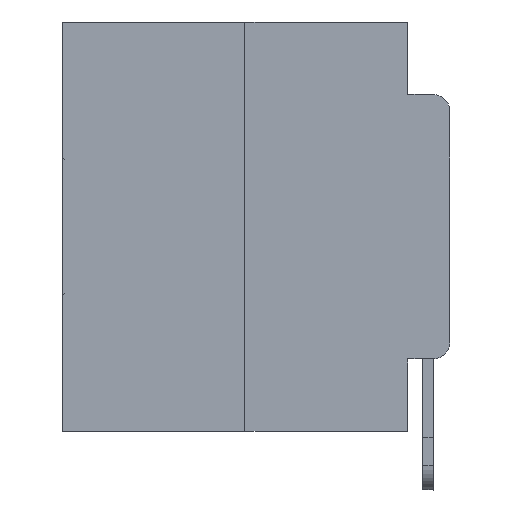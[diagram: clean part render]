
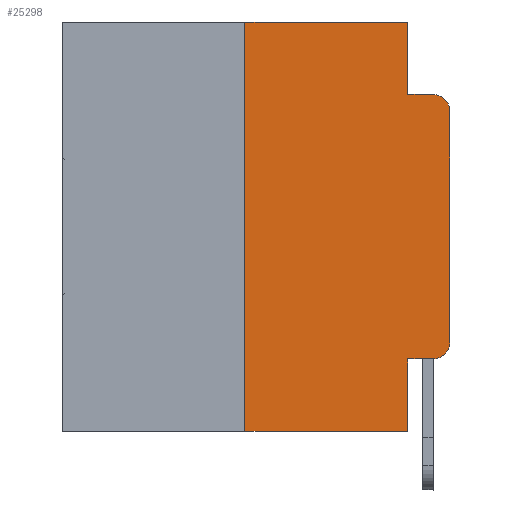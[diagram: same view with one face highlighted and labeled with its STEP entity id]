
A CAD part, left-side view. The second image highlights one B-rep face of the part: STEP entity #25298.
In plain terms, the highlighted planar face has unit normal (-1, 0, 0).
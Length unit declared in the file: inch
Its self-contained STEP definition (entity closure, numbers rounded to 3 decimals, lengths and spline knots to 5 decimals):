
#130 = VECTOR ( 'NONE', #13997, 39.37008 ) ;
#532 = ORIENTED_EDGE ( 'NONE', *, *, #11982, .T. ) ;
#886 = EDGE_CURVE ( 'NONE', #19352, #8026, #24660, .T. ) ;
#1176 = CARTESIAN_POINT ( 'NONE',  ( 0., 0.473, 0. ) ) ;
#1223 = CARTESIAN_POINT ( 'NONE',  ( 0., 0., -0.1085 ) ) ;
#1340 = LINE ( 'NONE', #13745, #18940 ) ;
#2053 = ORIENTED_EDGE ( 'NONE', *, *, #2154, .F. ) ;
#2087 = VECTOR ( 'NONE', #6164, 39.37008 ) ;
#2154 = EDGE_CURVE ( 'NONE', #3891, #13983, #21963, .T. ) ;
#2384 = ORIENTED_EDGE ( 'NONE', *, *, #26348, .F. ) ;
#3528 = DIRECTION ( 'NONE',  ( -1., 0., 0. ) ) ;
#3891 = VERTEX_POINT ( 'NONE', #13597 ) ;
#3935 = DIRECTION ( 'NONE',  ( 0., -1., 0. ) ) ;
#4432 = LINE ( 'NONE', #24332, #28053 ) ;
#5419 = ORIENTED_EDGE ( 'NONE', *, *, #17209, .F. ) ;
#6070 = CARTESIAN_POINT ( 'NONE',  ( 0., 0., 0. ) ) ;
#6164 = DIRECTION ( 'NONE',  ( 0., 0., 1. ) ) ;
#6978 = CARTESIAN_POINT ( 'NONE',  ( 0., 0.02, -0.4115 ) ) ;
#7017 = EDGE_CURVE ( 'NONE', #18324, #24548, #26638, .T. ) ;
#7060 = CARTESIAN_POINT ( 'NONE',  ( 0., 0.051, -0.0885 ) ) ;
#7067 = CARTESIAN_POINT ( 'NONE',  ( 0., 0.051, 0. ) ) ;
#8026 = VERTEX_POINT ( 'NONE', #6978 ) ;
#8273 = CARTESIAN_POINT ( 'NONE',  ( 0., 0.051, 0. ) ) ;
#8702 = ORIENTED_EDGE ( 'NONE', *, *, #23563, .T. ) ;
#9861 = CARTESIAN_POINT ( 'NONE',  ( 0., 0.02, -0.0885 ) ) ;
#9967 = ORIENTED_EDGE ( 'NONE', *, *, #7017, .T. ) ;
#10053 = VECTOR ( 'NONE', #12618, 39.37008 ) ;
#10339 = EDGE_CURVE ( 'NONE', #19352, #19735, #18447, .T. ) ;
#10655 = EDGE_LOOP ( 'NONE', ( #532, #9967, #29059, #2053, #5419, #2384, #21065, #13133, #23155, #8702 ) ) ;
#11982 = EDGE_CURVE ( 'NONE', #29237, #18324, #27941, .T. ) ;
#12618 = DIRECTION ( 'NONE',  ( 0., 0., 1. ) ) ;
#12788 = AXIS2_PLACEMENT_3D ( 'NONE', #14860, #3528, #26410 ) ;
#12840 = DIRECTION ( 'NONE',  ( 0., -1., 0. ) ) ;
#12904 = DIRECTION ( 'NONE',  ( 0., -1., 0. ) ) ;
#13133 = ORIENTED_EDGE ( 'NONE', *, *, #10339, .F. ) ;
#13396 = CARTESIAN_POINT ( 'NONE',  ( 0., 0.25, -0.5 ) ) ;
#13597 = CARTESIAN_POINT ( 'NONE',  ( 0., 0.051, 0. ) ) ;
#13680 = VERTEX_POINT ( 'NONE', #15110 ) ;
#13745 = CARTESIAN_POINT ( 'NONE',  ( 0., 0.473, -0.5 ) ) ;
#13842 = DIRECTION ( 'NONE',  ( 0., -1., 0. ) ) ;
#13864 = DIRECTION ( 'NONE',  ( 1., 0., 0. ) ) ;
#13967 = AXIS2_PLACEMENT_3D ( 'NONE', #22768, #13864, #25258 ) ;
#13983 = VERTEX_POINT ( 'NONE', #7060 ) ;
#13997 = DIRECTION ( 'NONE',  ( 0., 0., -1. ) ) ;
#14196 = EDGE_CURVE ( 'NONE', #13983, #24548, #4432, .T. ) ;
#14860 = CARTESIAN_POINT ( 'NONE',  ( 0., 0.02, -0.3915 ) ) ;
#15064 = CARTESIAN_POINT ( 'NONE',  ( 0., 0.051, -0.4115 ) ) ;
#15097 = CARTESIAN_POINT ( 'NONE',  ( 0., 0.25, 0. ) ) ;
#15110 = CARTESIAN_POINT ( 'NONE',  ( 0., 0.25, 0. ) ) ;
#15149 = VECTOR ( 'NONE', #29164, 39.37008 ) ;
#15243 = CARTESIAN_POINT ( 'NONE',  ( 0., 0.02, -0.1085 ) ) ;
#15351 = DIRECTION ( 'NONE',  ( 0., 0., -1. ) ) ;
#15655 = DIRECTION ( 'NONE',  ( -1., 0., 0. ) ) ;
#16658 = CARTESIAN_POINT ( 'NONE',  ( 0., 0.051, -0.4115 ) ) ;
#17209 = EDGE_CURVE ( 'NONE', #13680, #3891, #17599, .T. ) ;
#17599 = LINE ( 'NONE', #1176, #27919 ) ;
#17912 = FACE_OUTER_BOUND ( 'NONE', #10655, .T. ) ;
#18324 = VERTEX_POINT ( 'NONE', #1223 ) ;
#18358 = CIRCLE ( 'NONE', #12788, 0.02 ) ;
#18447 = LINE ( 'NONE', #7067, #130 ) ;
#18646 = EDGE_CURVE ( 'NONE', #20376, #19735, #1340, .T. ) ;
#18940 = VECTOR ( 'NONE', #13842, 39.37008 ) ;
#19345 = CARTESIAN_POINT ( 'NONE',  ( 0., 0., -0.3915 ) ) ;
#19352 = VERTEX_POINT ( 'NONE', #16658 ) ;
#19735 = VERTEX_POINT ( 'NONE', #24720 ) ;
#20376 = VERTEX_POINT ( 'NONE', #13396 ) ;
#20682 = PLANE ( 'NONE',  #13967 ) ;
#20736 = LINE ( 'NONE', #15097, #2087 ) ;
#21065 = ORIENTED_EDGE ( 'NONE', *, *, #18646, .T. ) ;
#21963 = LINE ( 'NONE', #8273, #15149 ) ;
#22768 = CARTESIAN_POINT ( 'NONE',  ( 0., 0.473, 0. ) ) ;
#23155 = ORIENTED_EDGE ( 'NONE', *, *, #886, .T. ) ;
#23563 = EDGE_CURVE ( 'NONE', #8026, #29237, #18358, .T. ) ;
#23707 = AXIS2_PLACEMENT_3D ( 'NONE', #15243, #15655, #15351 ) ;
#24332 = CARTESIAN_POINT ( 'NONE',  ( 0., 0.051, -0.0885 ) ) ;
#24548 = VERTEX_POINT ( 'NONE', #9861 ) ;
#24660 = LINE ( 'NONE', #15064, #29258 ) ;
#24720 = CARTESIAN_POINT ( 'NONE',  ( 0., 0.051, -0.5 ) ) ;
#25258 = DIRECTION ( 'NONE',  ( 0., 0., -1. ) ) ;
#25298 = ADVANCED_FACE ( 'NONE', ( #17912 ), #20682, .F. ) ;
#26348 = EDGE_CURVE ( 'NONE', #20376, #13680, #20736, .T. ) ;
#26410 = DIRECTION ( 'NONE',  ( 0., 0., -1. ) ) ;
#26638 = CIRCLE ( 'NONE', #23707, 0.02 ) ;
#27919 = VECTOR ( 'NONE', #12904, 39.37008 ) ;
#27941 = LINE ( 'NONE', #6070, #10053 ) ;
#28053 = VECTOR ( 'NONE', #12840, 39.37008 ) ;
#29059 = ORIENTED_EDGE ( 'NONE', *, *, #14196, .F. ) ;
#29164 = DIRECTION ( 'NONE',  ( 0., 0., -1. ) ) ;
#29237 = VERTEX_POINT ( 'NONE', #19345 ) ;
#29258 = VECTOR ( 'NONE', #3935, 39.37008 ) ;
